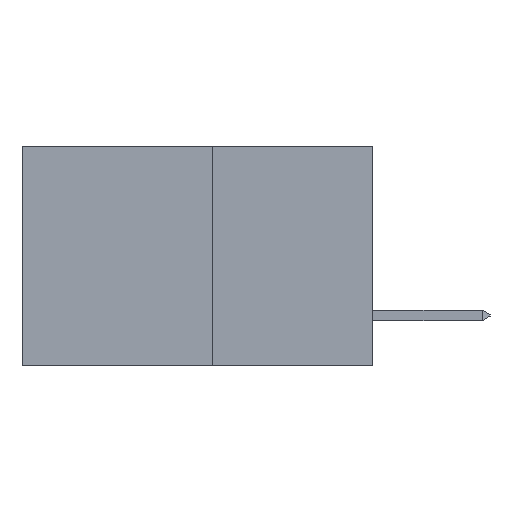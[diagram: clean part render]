
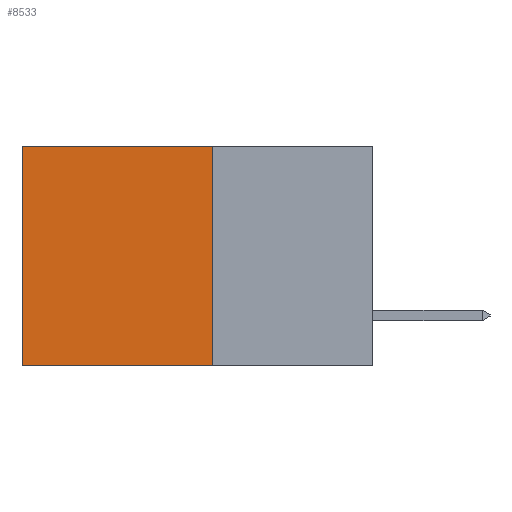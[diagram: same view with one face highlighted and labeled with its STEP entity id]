
A CAD part, left-side view. The second image highlights one B-rep face of the part: STEP entity #8533.
In plain terms, the highlighted planar face has unit normal (-1, 0, 0).
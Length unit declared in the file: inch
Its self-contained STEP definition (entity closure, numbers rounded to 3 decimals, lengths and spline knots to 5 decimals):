
#639 = LINE ( 'NONE', #12496, #4573 ) ;
#3116 = CARTESIAN_POINT ( 'NONE',  ( 0.277, 0.27, 0. ) ) ;
#3868 = LINE ( 'NONE', #5952, #16340 ) ;
#3917 = VERTEX_POINT ( 'NONE', #16362 ) ;
#4032 = VERTEX_POINT ( 'NONE', #15004 ) ;
#4254 = PLANE ( 'NONE',  #17826 ) ;
#4573 = VECTOR ( 'NONE', #6075, 39.37008 ) ;
#5320 = VECTOR ( 'NONE', #10528, 39.37008 ) ;
#5573 = ORIENTED_EDGE ( 'NONE', *, *, #11823, .T. ) ;
#5920 = DIRECTION ( 'NONE',  ( 1., 0., 0. ) ) ;
#5952 = CARTESIAN_POINT ( 'NONE',  ( 0.277, 0.59, -0.37 ) ) ;
#6075 = DIRECTION ( 'NONE',  ( 0., 1., 0. ) ) ;
#6161 = VERTEX_POINT ( 'NONE', #16562 ) ;
#7596 = DIRECTION ( 'NONE',  ( 0., 0., -1. ) ) ;
#7977 = ORIENTED_EDGE ( 'NONE', *, *, #18873, .F. ) ;
#8436 = ORIENTED_EDGE ( 'NONE', *, *, #12562, .T. ) ;
#8533 = ADVANCED_FACE ( 'NONE', ( #13446 ), #4254, .F. ) ;
#9052 = VERTEX_POINT ( 'NONE', #17185 ) ;
#9529 = ORIENTED_EDGE ( 'NONE', *, *, #12933, .F. ) ;
#10391 = EDGE_LOOP ( 'NONE', ( #5573, #7977, #9529, #8436 ) ) ;
#10528 = DIRECTION ( 'NONE',  ( 0., 0., -1. ) ) ;
#11823 = EDGE_CURVE ( 'NONE', #4032, #3917, #3868, .T. ) ;
#12491 = VECTOR ( 'NONE', #16144, 39.37008 ) ;
#12496 = CARTESIAN_POINT ( 'NONE',  ( 0.277, 0.27, -0.37 ) ) ;
#12562 = EDGE_CURVE ( 'NONE', #9052, #4032, #17771, .T. ) ;
#12933 = EDGE_CURVE ( 'NONE', #9052, #6161, #14447, .T. ) ;
#13446 = FACE_OUTER_BOUND ( 'NONE', #10391, .T. ) ;
#14447 = LINE ( 'NONE', #18653, #5320 ) ;
#15004 = CARTESIAN_POINT ( 'NONE',  ( 0.277, 0.59, 0. ) ) ;
#15628 = CARTESIAN_POINT ( 'NONE',  ( 0.277, 0.27, -0.37 ) ) ;
#16144 = DIRECTION ( 'NONE',  ( 0., 1., 0. ) ) ;
#16340 = VECTOR ( 'NONE', #7596, 39.37008 ) ;
#16362 = CARTESIAN_POINT ( 'NONE',  ( 0.277, 0.59, -0.37 ) ) ;
#16562 = CARTESIAN_POINT ( 'NONE',  ( 0.277, 0.27, -0.37 ) ) ;
#17185 = CARTESIAN_POINT ( 'NONE',  ( 0.277, 0.27, 0. ) ) ;
#17258 = DIRECTION ( 'NONE',  ( 0., 0., -1. ) ) ;
#17771 = LINE ( 'NONE', #3116, #12491 ) ;
#17826 = AXIS2_PLACEMENT_3D ( 'NONE', #15628, #5920, #17258 ) ;
#18653 = CARTESIAN_POINT ( 'NONE',  ( 0.277, 0.27, -0.37 ) ) ;
#18873 = EDGE_CURVE ( 'NONE', #6161, #3917, #639, .T. ) ;
